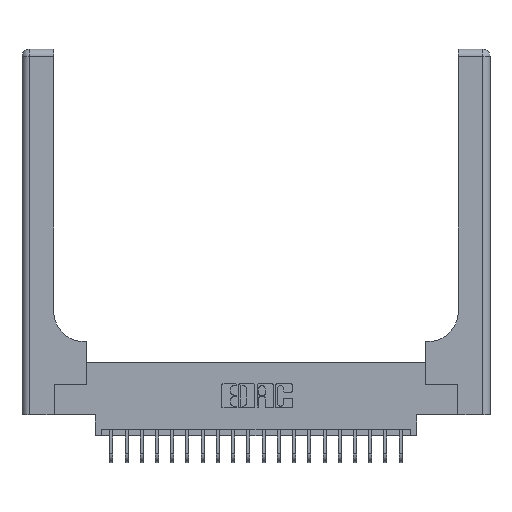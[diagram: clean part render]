
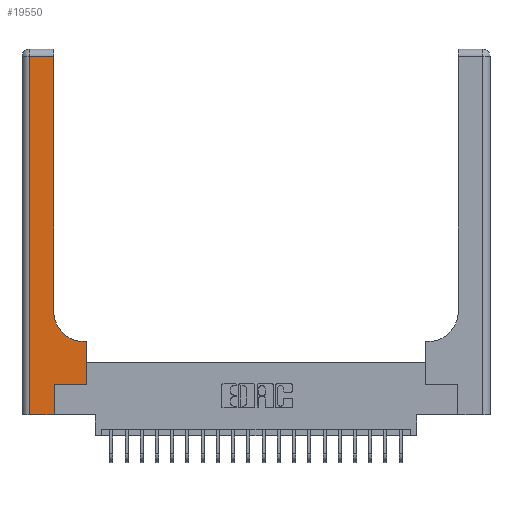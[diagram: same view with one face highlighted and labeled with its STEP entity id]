
A CAD part, top view. The second image highlights one B-rep face of the part: STEP entity #19550.
In plain terms, the highlighted planar face has unit normal (0, 0, 1).
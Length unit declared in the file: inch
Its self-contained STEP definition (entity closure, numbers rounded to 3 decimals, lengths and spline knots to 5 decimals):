
#146 = EDGE_CURVE ( 'NONE', #869, #4922, #2379, .T. ) ;
#436 = AXIS2_PLACEMENT_3D ( 'NONE', #17497, #8676, #8196 ) ;
#869 = VERTEX_POINT ( 'NONE', #21646 ) ;
#1572 = LINE ( 'NONE', #12631, #20900 ) ;
#1850 = EDGE_CURVE ( 'NONE', #2867, #4379, #1572, .T. ) ;
#2379 = LINE ( 'NONE', #14655, #17036 ) ;
#2403 = CARTESIAN_POINT ( 'NONE',  ( 0.265, 0., 0.37 ) ) ;
#2537 = CARTESIAN_POINT ( 'NONE',  ( 0.51, 0.6, 0.37 ) ) ;
#2707 = EDGE_CURVE ( 'NONE', #4922, #2867, #23085, .T. ) ;
#2722 = CARTESIAN_POINT ( 'NONE',  ( 0., 2.94, 0.37 ) ) ;
#2867 = VERTEX_POINT ( 'NONE', #2403 ) ;
#3184 = PLANE ( 'NONE',  #18748 ) ;
#3876 = ORIENTED_EDGE ( 'NONE', *, *, #17938, .T. ) ;
#4165 = VERTEX_POINT ( 'NONE', #14345 ) ;
#4322 = LINE ( 'NONE', #18868, #13578 ) ;
#4379 = VERTEX_POINT ( 'NONE', #16373 ) ;
#4563 = ORIENTED_EDGE ( 'NONE', *, *, #2707, .T. ) ;
#4631 = DIRECTION ( 'NONE',  ( -1., 0., 0. ) ) ;
#4922 = VERTEX_POINT ( 'NONE', #15541 ) ;
#4926 = CARTESIAN_POINT ( 'NONE',  ( 0.26, 0.85, 0.37 ) ) ;
#5098 = VERTEX_POINT ( 'NONE', #4926 ) ;
#6121 = LINE ( 'NONE', #13045, #7726 ) ;
#7023 = EDGE_CURVE ( 'NONE', #15995, #869, #15609, .T. ) ;
#7567 = DIRECTION ( 'NONE',  ( 1., 0., 0. ) ) ;
#7726 = VECTOR ( 'NONE', #7567, 39.37008 ) ;
#8196 = DIRECTION ( 'NONE',  ( 1., 0., 0. ) ) ;
#8301 = FACE_OUTER_BOUND ( 'NONE', #23434, .T. ) ;
#8541 = DIRECTION ( 'NONE',  ( -1., 0., 0. ) ) ;
#8676 = DIRECTION ( 'NONE',  ( 0., 0., -1. ) ) ;
#8804 = DIRECTION ( 'NONE',  ( -1., 0., 0. ) ) ;
#8934 = VERTEX_POINT ( 'NONE', #2537 ) ;
#9047 = EDGE_CURVE ( 'NONE', #13887, #4165, #4322, .T. ) ;
#9509 = VECTOR ( 'NONE', #16985, 39.37008 ) ;
#9786 = DIRECTION ( 'NONE',  ( 0., 1., 0. ) ) ;
#10559 = CARTESIAN_POINT ( 'NONE',  ( 0., 3., 0.37 ) ) ;
#10585 = LINE ( 'NONE', #17868, #20625 ) ;
#10706 = CIRCLE ( 'NONE', #436, 0.25 ) ;
#10846 = ORIENTED_EDGE ( 'NONE', *, *, #14490, .T. ) ;
#11531 = DIRECTION ( 'NONE',  ( 0., -1., 0. ) ) ;
#12337 = CARTESIAN_POINT ( 'NONE',  ( 0., 0., 0.37 ) ) ;
#12547 = ORIENTED_EDGE ( 'NONE', *, *, #19094, .T. ) ;
#12631 = CARTESIAN_POINT ( 'NONE',  ( 0.265, 0., 0.37 ) ) ;
#13045 = CARTESIAN_POINT ( 'NONE',  ( 0.265, 0.25, 0.37 ) ) ;
#13578 = VECTOR ( 'NONE', #9786, 39.37008 ) ;
#13887 = VERTEX_POINT ( 'NONE', #20478 ) ;
#14345 = CARTESIAN_POINT ( 'NONE',  ( 0.528, 0.6, 0.37 ) ) ;
#14490 = EDGE_CURVE ( 'NONE', #5098, #15995, #20792, .T. ) ;
#14527 = VECTOR ( 'NONE', #17597, 39.37008 ) ;
#14655 = CARTESIAN_POINT ( 'NONE',  ( 0.06, 3., 0.37 ) ) ;
#15541 = CARTESIAN_POINT ( 'NONE',  ( 0.06, 0., 0.37 ) ) ;
#15609 = LINE ( 'NONE', #2722, #18114 ) ;
#15948 = DIRECTION ( 'NONE',  ( 0., 0., -1. ) ) ;
#15995 = VERTEX_POINT ( 'NONE', #19573 ) ;
#16373 = CARTESIAN_POINT ( 'NONE',  ( 0.265, 0.25, 0.37 ) ) ;
#16966 = ORIENTED_EDGE ( 'NONE', *, *, #146, .T. ) ;
#16985 = DIRECTION ( 'NONE',  ( 0., 1., 0. ) ) ;
#17036 = VECTOR ( 'NONE', #11531, 39.37008 ) ;
#17054 = ORIENTED_EDGE ( 'NONE', *, *, #1850, .T. ) ;
#17337 = CARTESIAN_POINT ( 'NONE',  ( 0.26, 3., 0.37 ) ) ;
#17497 = CARTESIAN_POINT ( 'NONE',  ( 0.51, 0.85, 0.37 ) ) ;
#17564 = ORIENTED_EDGE ( 'NONE', *, *, #19789, .T. ) ;
#17597 = DIRECTION ( 'NONE',  ( 1., 0., 0. ) ) ;
#17868 = CARTESIAN_POINT ( 'NONE',  ( 0.26, 0.6, 0.37 ) ) ;
#17938 = EDGE_CURVE ( 'NONE', #8934, #5098, #10706, .T. ) ;
#18114 = VECTOR ( 'NONE', #4631, 39.37008 ) ;
#18125 = DIRECTION ( 'NONE',  ( 0., 1., 0. ) ) ;
#18748 = AXIS2_PLACEMENT_3D ( 'NONE', #10559, #15948, #8541 ) ;
#18868 = CARTESIAN_POINT ( 'NONE',  ( 0.528, 0.25, 0.37 ) ) ;
#19094 = EDGE_CURVE ( 'NONE', #4165, #8934, #10585, .T. ) ;
#19452 = ORIENTED_EDGE ( 'NONE', *, *, #9047, .T. ) ;
#19550 = ADVANCED_FACE ( 'NONE', ( #8301 ), #3184, .F. ) ;
#19573 = CARTESIAN_POINT ( 'NONE',  ( 0.26, 2.94, 0.37 ) ) ;
#19789 = EDGE_CURVE ( 'NONE', #4379, #13887, #6121, .T. ) ;
#20478 = CARTESIAN_POINT ( 'NONE',  ( 0.528, 0.25, 0.37 ) ) ;
#20625 = VECTOR ( 'NONE', #8804, 39.37008 ) ;
#20792 = LINE ( 'NONE', #17337, #9509 ) ;
#20900 = VECTOR ( 'NONE', #18125, 39.37008 ) ;
#21646 = CARTESIAN_POINT ( 'NONE',  ( 0.06, 2.94, 0.37 ) ) ;
#22910 = ORIENTED_EDGE ( 'NONE', *, *, #7023, .T. ) ;
#23085 = LINE ( 'NONE', #12337, #14527 ) ;
#23434 = EDGE_LOOP ( 'NONE', ( #10846, #22910, #16966, #4563, #17054, #17564, #19452, #12547, #3876 ) ) ;
